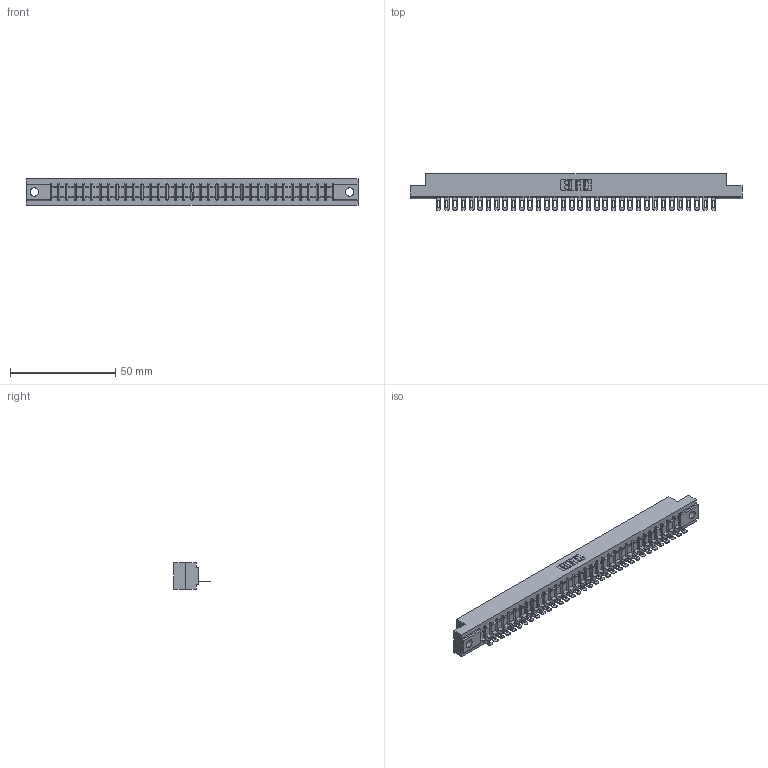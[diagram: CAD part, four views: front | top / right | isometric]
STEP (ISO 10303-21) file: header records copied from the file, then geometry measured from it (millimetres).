
FILE_DESCRIPTION (( 'STEP AP203' ), '1' );
FILE_NAME ('307-034-501-104.STEP', '2019-09-05T06:21:12', ( '' ), ( '' ), 'SwSTEP 2.0', 'SolidWorks 2016', '' );
FILE_SCHEMA (( 'CONFIG_CONTROL_DESIGN' ));
Length unit declared in the file: inch
Products named in the file (3): 307-290-002_501; 307-034-501-104; 307 Part_.156 Dia Mounting Holes
Assembly tree (35 placements, depth 2):
  307-034-501-104
    307 Part_.156 Dia Mounting Holes
    307-290-002_501  x34
Bounding box: 157.73 x 17.42 x 12.7 mm (x, y, z)
Volume: 16743.5 mm3; surface area: 20943 mm2
Topology: 35 solids, 35 shells, 2751 faces, 8451 edges, 5538 vertices
Faces by surface type: plane 1580, cylinder 1101, sphere 70
Entity records: 31346 total; most frequent: CARTESIAN_POINT 5290, ORIENTED_EDGE 5278, DIRECTION 5139, EDGE_CURVE 2639, LINE 2021, VECTOR 2021, VERTEX_POINT 1710, AXIS2_PLACEMENT_3D 1559
